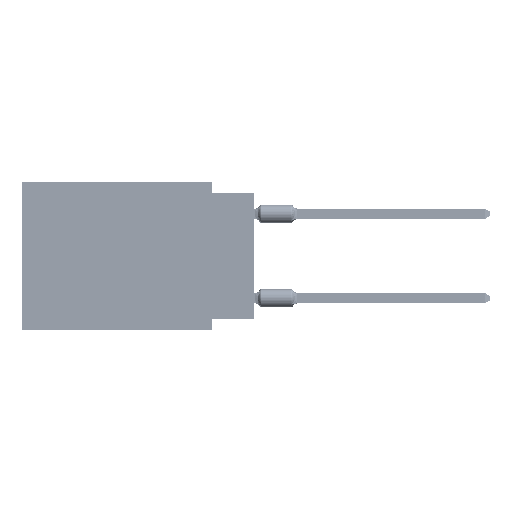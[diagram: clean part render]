
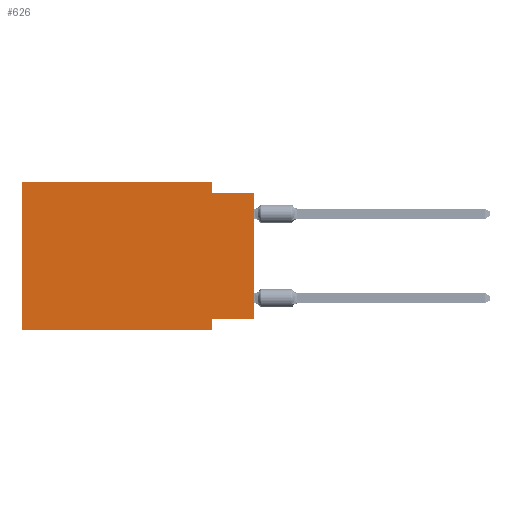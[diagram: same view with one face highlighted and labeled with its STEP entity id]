
A CAD part, left-side view. The second image highlights one B-rep face of the part: STEP entity #626.
In plain terms, the highlighted planar face has unit normal (-1, 0, 0).
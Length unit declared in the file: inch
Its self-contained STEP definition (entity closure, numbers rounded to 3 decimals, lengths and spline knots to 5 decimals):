
#626 = ADVANCED_FACE ( 'NONE', ( #4992 ), #81322, .F. ) ;
#1466 = DIRECTION ( 'NONE',  ( 0., 0., 1. ) ) ;
#3968 = ORIENTED_EDGE ( 'NONE', *, *, #43382, .F. ) ;
#4992 = FACE_OUTER_BOUND ( 'NONE', #19299, .T. ) ;
#6616 = CARTESIAN_POINT ( 'NONE',  ( 0., 0.55, 0. ) ) ;
#7799 = ORIENTED_EDGE ( 'NONE', *, *, #73177, .F. ) ;
#10767 = CARTESIAN_POINT ( 'NONE',  ( 0., 0.55, 0. ) ) ;
#13066 = CARTESIAN_POINT ( 'NONE',  ( 0., 0.55, 0. ) ) ;
#15972 = VERTEX_POINT ( 'NONE', #16538 ) ;
#16538 = CARTESIAN_POINT ( 'NONE',  ( 0., 0., -0.025 ) ) ;
#19299 = EDGE_LOOP ( 'NONE', ( #99362, #84727, #51281, #56487, #41703, #40111, #3968, #7799 ) ) ;
#21015 = VERTEX_POINT ( 'NONE', #77940 ) ;
#24626 = EDGE_CURVE ( 'NONE', #64171, #50372, #104809, .T. ) ;
#25188 = DIRECTION ( 'NONE',  ( 0., 0., -1. ) ) ;
#27694 = VECTOR ( 'NONE', #27937, 39.37008 ) ;
#27937 = DIRECTION ( 'NONE',  ( 0., -1., 0. ) ) ;
#29331 = DIRECTION ( 'NONE',  ( 0., -1., 0. ) ) ;
#31641 = CARTESIAN_POINT ( 'NONE',  ( 0., 0., -0.025 ) ) ;
#34251 = LINE ( 'NONE', #67971, #83011 ) ;
#35457 = LINE ( 'NONE', #37640, #39004 ) ;
#37640 = CARTESIAN_POINT ( 'NONE',  ( 0., 0.55, -0.35 ) ) ;
#39004 = VECTOR ( 'NONE', #29331, 39.37008 ) ;
#39306 = DIRECTION ( 'NONE',  ( 0., 0., -1. ) ) ;
#39959 = EDGE_CURVE ( 'NONE', #87521, #64171, #70608, .T. ) ;
#40111 = ORIENTED_EDGE ( 'NONE', *, *, #90396, .T. ) ;
#41703 = ORIENTED_EDGE ( 'NONE', *, *, #39959, .F. ) ;
#43207 = VECTOR ( 'NONE', #55970, 39.37008 ) ;
#43382 = EDGE_CURVE ( 'NONE', #101185, #60270, #76169, .T. ) ;
#43561 = LINE ( 'NONE', #77251, #57669 ) ;
#47192 = CARTESIAN_POINT ( 'NONE',  ( 0., 0., -0.325 ) ) ;
#47614 = DIRECTION ( 'NONE',  ( 1., 0., 0. ) ) ;
#50372 = VERTEX_POINT ( 'NONE', #98761 ) ;
#51281 = ORIENTED_EDGE ( 'NONE', *, *, #53068, .F. ) ;
#53068 = EDGE_CURVE ( 'NONE', #50372, #21015, #77154, .T. ) ;
#55664 = DIRECTION ( 'NONE',  ( 0., 0., 1. ) ) ;
#55970 = DIRECTION ( 'NONE',  ( 0., -1., 0. ) ) ;
#56487 = ORIENTED_EDGE ( 'NONE', *, *, #24626, .F. ) ;
#57669 = VECTOR ( 'NONE', #1466, 39.37008 ) ;
#60270 = VERTEX_POINT ( 'NONE', #90737 ) ;
#61084 = AXIS2_PLACEMENT_3D ( 'NONE', #6616, #47614, #39306 ) ;
#64171 = VERTEX_POINT ( 'NONE', #77393 ) ;
#66901 = CARTESIAN_POINT ( 'NONE',  ( 0., 0.55, -0.35 ) ) ;
#67450 = EDGE_CURVE ( 'NONE', #107911, #15972, #43561, .T. ) ;
#67881 = CARTESIAN_POINT ( 'NONE',  ( 0., 0.1, -0.35 ) ) ;
#67971 = CARTESIAN_POINT ( 'NONE',  ( 0., 0., -0.325 ) ) ;
#70608 = LINE ( 'NONE', #13066, #95507 ) ;
#72567 = LINE ( 'NONE', #31641, #43207 ) ;
#73177 = EDGE_CURVE ( 'NONE', #107911, #101185, #34251, .T. ) ;
#74893 = VECTOR ( 'NONE', #101609, 39.37008 ) ;
#76169 = LINE ( 'NONE', #67881, #74893 ) ;
#77154 = LINE ( 'NONE', #102595, #79639 ) ;
#77251 = CARTESIAN_POINT ( 'NONE',  ( 0., 0., 0. ) ) ;
#77393 = CARTESIAN_POINT ( 'NONE',  ( 0., 0.55, 0. ) ) ;
#77940 = CARTESIAN_POINT ( 'NONE',  ( 0., 0.1, -0.025 ) ) ;
#79639 = VECTOR ( 'NONE', #25188, 39.37008 ) ;
#81322 = PLANE ( 'NONE',  #61084 ) ;
#83011 = VECTOR ( 'NONE', #98167, 39.37008 ) ;
#84727 = ORIENTED_EDGE ( 'NONE', *, *, #106785, .F. ) ;
#87521 = VERTEX_POINT ( 'NONE', #66901 ) ;
#90396 = EDGE_CURVE ( 'NONE', #87521, #60270, #35457, .T. ) ;
#90737 = CARTESIAN_POINT ( 'NONE',  ( 0., 0.1, -0.35 ) ) ;
#92946 = CARTESIAN_POINT ( 'NONE',  ( 0., 0.1, -0.325 ) ) ;
#95507 = VECTOR ( 'NONE', #55664, 39.37008 ) ;
#98167 = DIRECTION ( 'NONE',  ( 0., 1., 0. ) ) ;
#98761 = CARTESIAN_POINT ( 'NONE',  ( 0., 0.1, 0. ) ) ;
#99362 = ORIENTED_EDGE ( 'NONE', *, *, #67450, .T. ) ;
#101185 = VERTEX_POINT ( 'NONE', #92946 ) ;
#101609 = DIRECTION ( 'NONE',  ( 0., 0., -1. ) ) ;
#102595 = CARTESIAN_POINT ( 'NONE',  ( 0., 0.1, 0. ) ) ;
#104809 = LINE ( 'NONE', #10767, #27694 ) ;
#106785 = EDGE_CURVE ( 'NONE', #21015, #15972, #72567, .T. ) ;
#107911 = VERTEX_POINT ( 'NONE', #47192 ) ;
